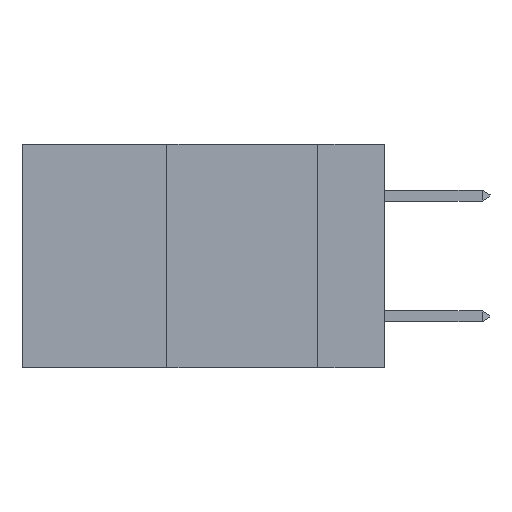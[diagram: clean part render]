
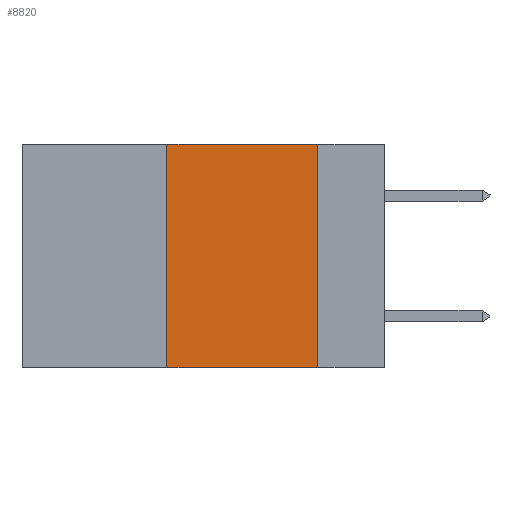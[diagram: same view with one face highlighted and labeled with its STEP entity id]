
A CAD part, left-side view. The second image highlights one B-rep face of the part: STEP entity #8820.
In plain terms, the highlighted planar face has unit normal (-1, 0, 0).
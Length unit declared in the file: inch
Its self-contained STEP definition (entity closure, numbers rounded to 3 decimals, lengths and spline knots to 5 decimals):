
#2466 = LINE ( 'NONE', #6916, #34042 ) ;
#5065 = LINE ( 'NONE', #10869, #42998 ) ;
#6386 = ORIENTED_EDGE ( 'NONE', *, *, #25318, .T. ) ;
#6916 = CARTESIAN_POINT ( 'NONE',  ( 0., 0.6, 0. ) ) ;
#7125 = CARTESIAN_POINT ( 'NONE',  ( 0., 0.6, 0. ) ) ;
#8457 = CARTESIAN_POINT ( 'NONE',  ( 0., 0.36, -0.37 ) ) ;
#8820 = ADVANCED_FACE ( 'NONE', ( #11019 ), #30845, .F. ) ;
#8995 = VERTEX_POINT ( 'NONE', #17985 ) ;
#9690 = DIRECTION ( 'NONE',  ( 0., 0., 1. ) ) ;
#9752 = VERTEX_POINT ( 'NONE', #41137 ) ;
#10105 = EDGE_CURVE ( 'NONE', #14891, #33277, #30436, .T. ) ;
#10775 = EDGE_LOOP ( 'NONE', ( #40637, #28646, #37991, #6386 ) ) ;
#10869 = CARTESIAN_POINT ( 'NONE',  ( 0., 0.11, 0. ) ) ;
#11019 = FACE_OUTER_BOUND ( 'NONE', #10775, .T. ) ;
#11217 = EDGE_CURVE ( 'NONE', #33277, #8995, #2466, .T. ) ;
#11242 = CARTESIAN_POINT ( 'NONE',  ( 0., 0.6, -0.37 ) ) ;
#11681 = DIRECTION ( 'NONE',  ( 0., -1., 0. ) ) ;
#12761 = VECTOR ( 'NONE', #11681, 39.37008 ) ;
#14891 = VERTEX_POINT ( 'NONE', #8457 ) ;
#16442 = EDGE_CURVE ( 'NONE', #8995, #9752, #5065, .T. ) ;
#17985 = CARTESIAN_POINT ( 'NONE',  ( 0., 0.11, 0. ) ) ;
#21749 = LINE ( 'NONE', #11242, #12761 ) ;
#23575 = VECTOR ( 'NONE', #9690, 39.37008 ) ;
#23869 = DIRECTION ( 'NONE',  ( 0., 0., -1. ) ) ;
#25318 = EDGE_CURVE ( 'NONE', #14891, #9752, #21749, .T. ) ;
#26787 = DIRECTION ( 'NONE',  ( 0., -1., 0. ) ) ;
#28027 = AXIS2_PLACEMENT_3D ( 'NONE', #7125, #34661, #38046 ) ;
#28646 = ORIENTED_EDGE ( 'NONE', *, *, #11217, .F. ) ;
#30436 = LINE ( 'NONE', #33443, #23575 ) ;
#30845 = PLANE ( 'NONE',  #28027 ) ;
#33277 = VERTEX_POINT ( 'NONE', #41402 ) ;
#33443 = CARTESIAN_POINT ( 'NONE',  ( 0., 0.36, 0. ) ) ;
#34042 = VECTOR ( 'NONE', #26787, 39.37008 ) ;
#34661 = DIRECTION ( 'NONE',  ( 1., 0., 0. ) ) ;
#37991 = ORIENTED_EDGE ( 'NONE', *, *, #10105, .F. ) ;
#38046 = DIRECTION ( 'NONE',  ( 0., 0., -1. ) ) ;
#40637 = ORIENTED_EDGE ( 'NONE', *, *, #16442, .F. ) ;
#41137 = CARTESIAN_POINT ( 'NONE',  ( 0., 0.11, -0.37 ) ) ;
#41402 = CARTESIAN_POINT ( 'NONE',  ( 0., 0.36, 0. ) ) ;
#42998 = VECTOR ( 'NONE', #23869, 39.37008 ) ;
